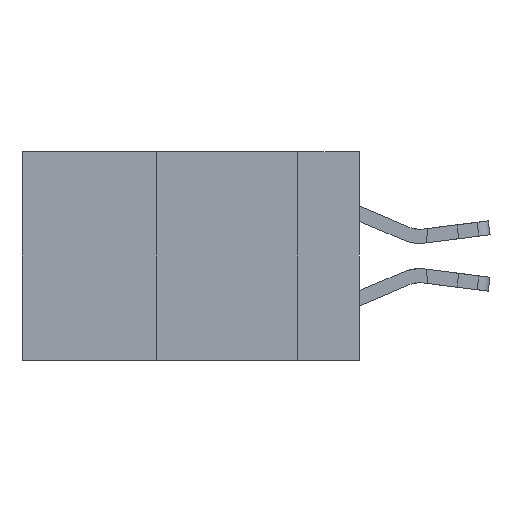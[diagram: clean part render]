
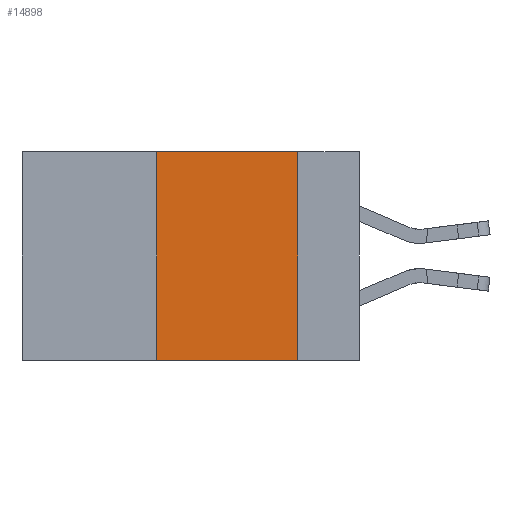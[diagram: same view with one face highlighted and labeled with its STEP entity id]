
A CAD part, left-side view. The second image highlights one B-rep face of the part: STEP entity #14898.
In plain terms, the highlighted planar face has unit normal (-1, 0, 0).
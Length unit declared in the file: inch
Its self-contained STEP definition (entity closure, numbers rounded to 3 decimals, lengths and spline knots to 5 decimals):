
#1113 = CARTESIAN_POINT ( 'NONE',  ( 0., 0.36, 0. ) ) ;
#1449 = VECTOR ( 'NONE', #31557, 39.37008 ) ;
#1514 = FACE_OUTER_BOUND ( 'NONE', #16420, .T. ) ;
#2063 = EDGE_CURVE ( 'NONE', #22661, #15962, #9815, .T. ) ;
#2122 = LINE ( 'NONE', #21712, #20471 ) ;
#4790 = VECTOR ( 'NONE', #22219, 39.37008 ) ;
#4828 = EDGE_CURVE ( 'NONE', #22661, #19235, #28174, .T. ) ;
#6426 = PLANE ( 'NONE',  #14353 ) ;
#9368 = DIRECTION ( 'NONE',  ( 0., -1., 0. ) ) ;
#9809 = VECTOR ( 'NONE', #9368, 39.37008 ) ;
#9815 = LINE ( 'NONE', #1113, #1449 ) ;
#10977 = ORIENTED_EDGE ( 'NONE', *, *, #24744, .F. ) ;
#12095 = LINE ( 'NONE', #17540, #9809 ) ;
#12269 = ORIENTED_EDGE ( 'NONE', *, *, #2063, .F. ) ;
#12853 = ORIENTED_EDGE ( 'NONE', *, *, #17156, .F. ) ;
#14353 = AXIS2_PLACEMENT_3D ( 'NONE', #22758, #33798, #20029 ) ;
#14855 = ORIENTED_EDGE ( 'NONE', *, *, #4828, .T. ) ;
#14898 = ADVANCED_FACE ( 'NONE', ( #1514 ), #6426, .F. ) ;
#15962 = VERTEX_POINT ( 'NONE', #22583 ) ;
#16420 = EDGE_LOOP ( 'NONE', ( #10977, #12853, #12269, #14855 ) ) ;
#17156 = EDGE_CURVE ( 'NONE', #15962, #27278, #12095, .T. ) ;
#17540 = CARTESIAN_POINT ( 'NONE',  ( 0., 0.6, 0. ) ) ;
#19235 = VERTEX_POINT ( 'NONE', #22363 ) ;
#20029 = DIRECTION ( 'NONE',  ( 0., 0., -1. ) ) ;
#20471 = VECTOR ( 'NONE', #27146, 39.37008 ) ;
#21712 = CARTESIAN_POINT ( 'NONE',  ( 0., 0.11, 0. ) ) ;
#22219 = DIRECTION ( 'NONE',  ( 0., -1., 0. ) ) ;
#22363 = CARTESIAN_POINT ( 'NONE',  ( 0., 0.11, -0.37 ) ) ;
#22583 = CARTESIAN_POINT ( 'NONE',  ( 0., 0.36, 0. ) ) ;
#22661 = VERTEX_POINT ( 'NONE', #30463 ) ;
#22758 = CARTESIAN_POINT ( 'NONE',  ( 0., 0.6, 0. ) ) ;
#24744 = EDGE_CURVE ( 'NONE', #27278, #19235, #2122, .T. ) ;
#27146 = DIRECTION ( 'NONE',  ( 0., 0., -1. ) ) ;
#27278 = VERTEX_POINT ( 'NONE', #32824 ) ;
#28174 = LINE ( 'NONE', #31062, #4790 ) ;
#30463 = CARTESIAN_POINT ( 'NONE',  ( 0., 0.36, -0.37 ) ) ;
#31062 = CARTESIAN_POINT ( 'NONE',  ( 0., 0.6, -0.37 ) ) ;
#31557 = DIRECTION ( 'NONE',  ( 0., 0., 1. ) ) ;
#32824 = CARTESIAN_POINT ( 'NONE',  ( 0., 0.11, 0. ) ) ;
#33798 = DIRECTION ( 'NONE',  ( 1., 0., 0. ) ) ;
